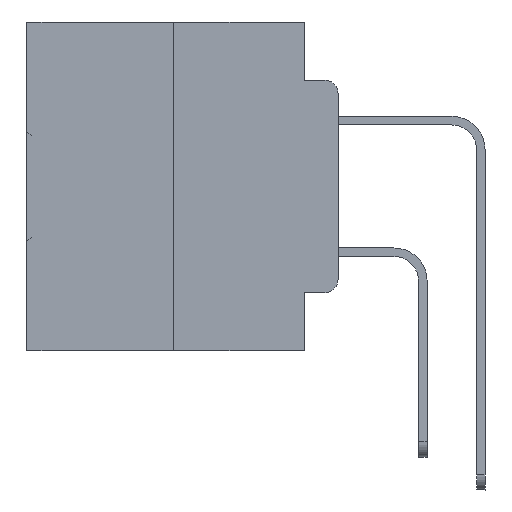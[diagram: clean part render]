
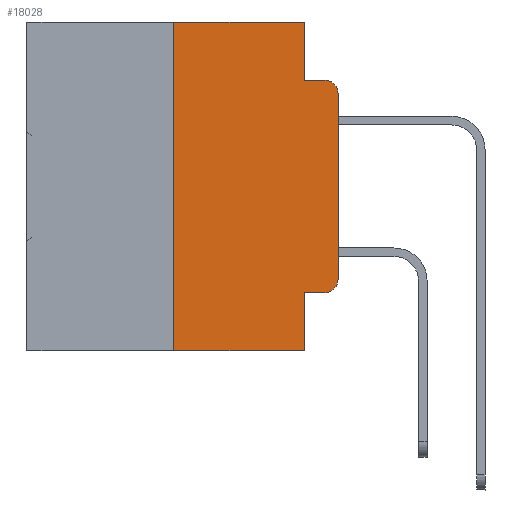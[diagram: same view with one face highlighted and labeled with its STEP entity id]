
A CAD part, left-side view. The second image highlights one B-rep face of the part: STEP entity #18028.
In plain terms, the highlighted planar face has unit normal (-1, 0, 0).
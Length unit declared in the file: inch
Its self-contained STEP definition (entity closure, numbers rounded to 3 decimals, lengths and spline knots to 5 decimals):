
#386 = LINE ( 'NONE', #3119, #30444 ) ;
#486 = AXIS2_PLACEMENT_3D ( 'NONE', #20343, #6650, #9006 ) ;
#911 = CARTESIAN_POINT ( 'NONE',  ( 0., 0.051, -0.0885 ) ) ;
#1505 = CARTESIAN_POINT ( 'NONE',  ( 0., 0.051, 0. ) ) ;
#2892 = ORIENTED_EDGE ( 'NONE', *, *, #30672, .F. ) ;
#2946 = DIRECTION ( 'NONE',  ( 0., 0., 1. ) ) ;
#2958 = CARTESIAN_POINT ( 'NONE',  ( 0., 0.051, -0.0885 ) ) ;
#3119 = CARTESIAN_POINT ( 'NONE',  ( 0., 0.25, 0. ) ) ;
#3433 = VECTOR ( 'NONE', #18732, 39.37008 ) ;
#3902 = ORIENTED_EDGE ( 'NONE', *, *, #35053, .F. ) ;
#4386 = AXIS2_PLACEMENT_3D ( 'NONE', #23485, #18228, #34365 ) ;
#5473 = VECTOR ( 'NONE', #34189, 39.37008 ) ;
#5846 = ORIENTED_EDGE ( 'NONE', *, *, #9544, .T. ) ;
#6199 = VERTEX_POINT ( 'NONE', #19361 ) ;
#6650 = DIRECTION ( 'NONE',  ( 1., 0., 0. ) ) ;
#6714 = VECTOR ( 'NONE', #21666, 39.37008 ) ;
#7015 = ORIENTED_EDGE ( 'NONE', *, *, #34869, .T. ) ;
#7486 = CARTESIAN_POINT ( 'NONE',  ( 0., 0.02, -0.3915 ) ) ;
#7895 = CARTESIAN_POINT ( 'NONE',  ( 0., 0.051, -0.5 ) ) ;
#8135 = EDGE_CURVE ( 'NONE', #27844, #11126, #14122, .T. ) ;
#8177 = ORIENTED_EDGE ( 'NONE', *, *, #16545, .F. ) ;
#8697 = CARTESIAN_POINT ( 'NONE',  ( 0., 0.25, 0. ) ) ;
#8910 = LINE ( 'NONE', #25841, #23255 ) ;
#8946 = VERTEX_POINT ( 'NONE', #11112 ) ;
#8991 = ORIENTED_EDGE ( 'NONE', *, *, #19069, .T. ) ;
#9006 = DIRECTION ( 'NONE',  ( 0., 0., -1. ) ) ;
#9544 = EDGE_CURVE ( 'NONE', #29826, #11126, #8910, .T. ) ;
#10139 = CARTESIAN_POINT ( 'NONE',  ( 0., 0., 0. ) ) ;
#10165 = CIRCLE ( 'NONE', #4386, 0.02 ) ;
#10716 = DIRECTION ( 'NONE',  ( 0., 0., -1. ) ) ;
#11112 = CARTESIAN_POINT ( 'NONE',  ( 0., 0., -0.1085 ) ) ;
#11126 = VERTEX_POINT ( 'NONE', #7895 ) ;
#11237 = CARTESIAN_POINT ( 'NONE',  ( 0., 0.051, 0. ) ) ;
#12232 = CARTESIAN_POINT ( 'NONE',  ( 0., 0.473, 0. ) ) ;
#13359 = LINE ( 'NONE', #10139, #6714 ) ;
#14122 = LINE ( 'NONE', #11237, #16043 ) ;
#14129 = DIRECTION ( 'NONE',  ( 0., -1., 0. ) ) ;
#14785 = VERTEX_POINT ( 'NONE', #31463 ) ;
#15962 = CARTESIAN_POINT ( 'NONE',  ( 0., 0.25, -0.5 ) ) ;
#16043 = VECTOR ( 'NONE', #31110, 39.37008 ) ;
#16545 = EDGE_CURVE ( 'NONE', #16635, #21434, #22113, .T. ) ;
#16635 = VERTEX_POINT ( 'NONE', #1505 ) ;
#17341 = LINE ( 'NONE', #911, #5473 ) ;
#17454 = PLANE ( 'NONE',  #486 ) ;
#17623 = LINE ( 'NONE', #12232, #30990 ) ;
#18028 = ADVANCED_FACE ( 'NONE', ( #31032 ), #17454, .F. ) ;
#18228 = DIRECTION ( 'NONE',  ( -1., 0., 0. ) ) ;
#18732 = DIRECTION ( 'NONE',  ( 0., -1., 0. ) ) ;
#18809 = VERTEX_POINT ( 'NONE', #8697 ) ;
#19069 = EDGE_CURVE ( 'NONE', #27844, #6199, #24174, .T. ) ;
#19361 = CARTESIAN_POINT ( 'NONE',  ( 0., 0.02, -0.4115 ) ) ;
#20336 = DIRECTION ( 'NONE',  ( 0., -1., 0. ) ) ;
#20343 = CARTESIAN_POINT ( 'NONE',  ( 0., 0.473, 0. ) ) ;
#21434 = VERTEX_POINT ( 'NONE', #2958 ) ;
#21666 = DIRECTION ( 'NONE',  ( 0., 0., 1. ) ) ;
#22113 = LINE ( 'NONE', #30080, #24109 ) ;
#22372 = CARTESIAN_POINT ( 'NONE',  ( 0., 0.051, -0.4115 ) ) ;
#23255 = VECTOR ( 'NONE', #14129, 39.37008 ) ;
#23485 = CARTESIAN_POINT ( 'NONE',  ( 0., 0.02, -0.1085 ) ) ;
#23641 = CARTESIAN_POINT ( 'NONE',  ( 0., 0.051, -0.4115 ) ) ;
#24109 = VECTOR ( 'NONE', #32995, 39.37008 ) ;
#24174 = LINE ( 'NONE', #23641, #3433 ) ;
#24899 = VERTEX_POINT ( 'NONE', #34677 ) ;
#25422 = ORIENTED_EDGE ( 'NONE', *, *, #32268, .T. ) ;
#25795 = CIRCLE ( 'NONE', #34515, 0.02 ) ;
#25841 = CARTESIAN_POINT ( 'NONE',  ( 0., 0.473, -0.5 ) ) ;
#27710 = ORIENTED_EDGE ( 'NONE', *, *, #8135, .F. ) ;
#27844 = VERTEX_POINT ( 'NONE', #22372 ) ;
#28627 = ORIENTED_EDGE ( 'NONE', *, *, #32034, .T. ) ;
#28833 = ORIENTED_EDGE ( 'NONE', *, *, #34401, .F. ) ;
#29826 = VERTEX_POINT ( 'NONE', #15962 ) ;
#30080 = CARTESIAN_POINT ( 'NONE',  ( 0., 0.051, 0. ) ) ;
#30444 = VECTOR ( 'NONE', #2946, 39.37008 ) ;
#30672 = EDGE_CURVE ( 'NONE', #21434, #24899, #17341, .T. ) ;
#30990 = VECTOR ( 'NONE', #20336, 39.37008 ) ;
#31032 = FACE_OUTER_BOUND ( 'NONE', #33782, .T. ) ;
#31110 = DIRECTION ( 'NONE',  ( 0., 0., -1. ) ) ;
#31463 = CARTESIAN_POINT ( 'NONE',  ( 0., 0., -0.3915 ) ) ;
#32034 = EDGE_CURVE ( 'NONE', #14785, #8946, #13359, .T. ) ;
#32268 = EDGE_CURVE ( 'NONE', #8946, #24899, #10165, .T. ) ;
#32995 = DIRECTION ( 'NONE',  ( 0., 0., -1. ) ) ;
#33782 = EDGE_LOOP ( 'NONE', ( #28627, #25422, #2892, #8177, #28833, #3902, #5846, #27710, #8991, #7015 ) ) ;
#34189 = DIRECTION ( 'NONE',  ( 0., -1., 0. ) ) ;
#34365 = DIRECTION ( 'NONE',  ( 0., 0., -1. ) ) ;
#34401 = EDGE_CURVE ( 'NONE', #18809, #16635, #17623, .T. ) ;
#34515 = AXIS2_PLACEMENT_3D ( 'NONE', #7486, #35319, #10716 ) ;
#34677 = CARTESIAN_POINT ( 'NONE',  ( 0., 0.02, -0.0885 ) ) ;
#34869 = EDGE_CURVE ( 'NONE', #6199, #14785, #25795, .T. ) ;
#35053 = EDGE_CURVE ( 'NONE', #29826, #18809, #386, .T. ) ;
#35319 = DIRECTION ( 'NONE',  ( -1., 0., 0. ) ) ;
